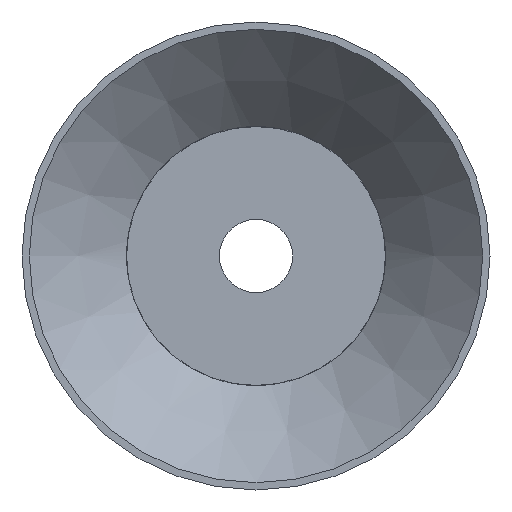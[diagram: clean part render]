
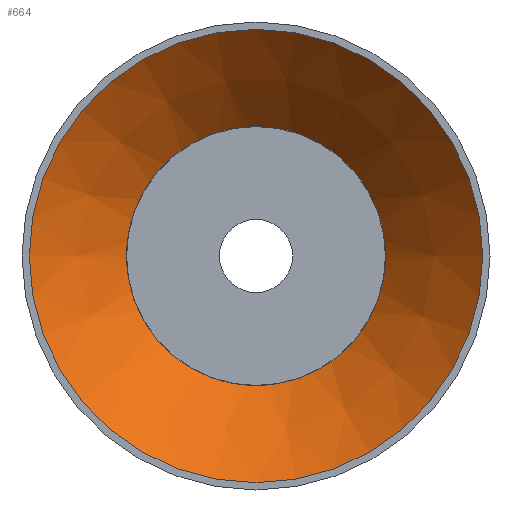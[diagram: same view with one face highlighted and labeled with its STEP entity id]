
A CAD part, front view. The second image highlights one B-rep face of the part: STEP entity #664.
In plain terms, the highlighted conical face has half-angle 43.531 degrees and reference radius 30.924 mm.
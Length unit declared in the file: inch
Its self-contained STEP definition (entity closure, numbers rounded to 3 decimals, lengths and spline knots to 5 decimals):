
#115=FACE_OUTER_BOUND('',#147,.T.);
#147=EDGE_LOOP('',(#434,#435,#436,#437,#438,#439,#440,#441,#442,#443,#444,
#445,#446));
#182=LINE('',#888,#196);
#196=VECTOR('',#768,1.2175);
#210=CIRCLE('',#711,1.55);
#211=CIRCLE('',#712,0.885);
#212=CIRCLE('',#713,0.885);
#213=CIRCLE('',#714,0.885);
#214=CIRCLE('',#715,0.885);
#215=CIRCLE('',#716,0.885);
#216=CIRCLE('',#717,0.885);
#217=CIRCLE('',#718,0.885);
#218=CIRCLE('',#719,0.885);
#219=CIRCLE('',#720,0.885);
#220=CIRCLE('',#721,1.55);
#243=VERTEX_POINT('',#884);
#244=VERTEX_POINT('',#885);
#245=VERTEX_POINT('',#887);
#246=VERTEX_POINT('',#889);
#247=VERTEX_POINT('',#891);
#248=VERTEX_POINT('',#893);
#249=VERTEX_POINT('',#895);
#250=VERTEX_POINT('',#897);
#251=VERTEX_POINT('',#899);
#252=VERTEX_POINT('',#901);
#253=VERTEX_POINT('',#903);
#320=EDGE_CURVE('',#243,#244,#210,.T.);
#321=EDGE_CURVE('',#244,#245,#182,.T.);
#322=EDGE_CURVE('',#246,#245,#211,.T.);
#323=EDGE_CURVE('',#247,#246,#212,.T.);
#324=EDGE_CURVE('',#248,#247,#213,.T.);
#325=EDGE_CURVE('',#249,#248,#214,.T.);
#326=EDGE_CURVE('',#250,#249,#215,.T.);
#327=EDGE_CURVE('',#251,#250,#216,.T.);
#328=EDGE_CURVE('',#252,#251,#217,.T.);
#329=EDGE_CURVE('',#253,#252,#218,.T.);
#330=EDGE_CURVE('',#245,#253,#219,.T.);
#331=EDGE_CURVE('',#244,#243,#220,.T.);
#434=ORIENTED_EDGE('',*,*,#320,.T.);
#435=ORIENTED_EDGE('',*,*,#321,.T.);
#436=ORIENTED_EDGE('',*,*,#322,.F.);
#437=ORIENTED_EDGE('',*,*,#323,.F.);
#438=ORIENTED_EDGE('',*,*,#324,.F.);
#439=ORIENTED_EDGE('',*,*,#325,.F.);
#440=ORIENTED_EDGE('',*,*,#326,.F.);
#441=ORIENTED_EDGE('',*,*,#327,.F.);
#442=ORIENTED_EDGE('',*,*,#328,.F.);
#443=ORIENTED_EDGE('',*,*,#329,.F.);
#444=ORIENTED_EDGE('',*,*,#330,.F.);
#445=ORIENTED_EDGE('',*,*,#321,.F.);
#446=ORIENTED_EDGE('',*,*,#331,.T.);
#662=CONICAL_SURFACE('',#710,1.2175,0.76);
#664=ADVANCED_FACE('',(#115),#662,.F.);
#710=AXIS2_PLACEMENT_3D('',#883,#764,#765);
#711=AXIS2_PLACEMENT_3D('',#886,#766,#767);
#712=AXIS2_PLACEMENT_3D('',#890,#769,#770);
#713=AXIS2_PLACEMENT_3D('',#892,#771,#772);
#714=AXIS2_PLACEMENT_3D('',#894,#773,#774);
#715=AXIS2_PLACEMENT_3D('',#896,#775,#776);
#716=AXIS2_PLACEMENT_3D('',#898,#777,#778);
#717=AXIS2_PLACEMENT_3D('',#900,#779,#780);
#718=AXIS2_PLACEMENT_3D('',#902,#781,#782);
#719=AXIS2_PLACEMENT_3D('',#904,#783,#784);
#720=AXIS2_PLACEMENT_3D('',#905,#785,#786);
#721=AXIS2_PLACEMENT_3D('',#906,#787,#788);
#764=DIRECTION('center_axis',(0.,-1.,0.));
#765=DIRECTION('ref_axis',(1.,0.,0.));
#766=DIRECTION('center_axis',(0.,-1.,0.));
#767=DIRECTION('ref_axis',(1.,0.,0.));
#768=DIRECTION('',(0.689,0.725,0.));
#769=DIRECTION('center_axis',(0.,-1.,0.));
#770=DIRECTION('ref_axis',(1.,0.,0.));
#771=DIRECTION('center_axis',(0.,-1.,0.));
#772=DIRECTION('ref_axis',(1.,0.,0.));
#773=DIRECTION('center_axis',(0.,-1.,0.));
#774=DIRECTION('ref_axis',(1.,0.,0.));
#775=DIRECTION('center_axis',(0.,-1.,0.));
#776=DIRECTION('ref_axis',(1.,0.,0.));
#777=DIRECTION('center_axis',(0.,-1.,0.));
#778=DIRECTION('ref_axis',(1.,0.,0.));
#779=DIRECTION('center_axis',(0.,-1.,0.));
#780=DIRECTION('ref_axis',(1.,0.,0.));
#781=DIRECTION('center_axis',(0.,-1.,0.));
#782=DIRECTION('ref_axis',(1.,0.,0.));
#783=DIRECTION('center_axis',(0.,-1.,0.));
#784=DIRECTION('ref_axis',(1.,0.,0.));
#785=DIRECTION('center_axis',(0.,-1.,0.));
#786=DIRECTION('ref_axis',(1.,0.,0.));
#787=DIRECTION('center_axis',(0.,-1.,0.));
#788=DIRECTION('ref_axis',(1.,0.,0.));
#883=CARTESIAN_POINT('Origin',(0.,0.35,0.));
#884=CARTESIAN_POINT('',(1.55,0.,0.));
#885=CARTESIAN_POINT('',(-1.55,0.,0.));
#886=CARTESIAN_POINT('Origin',(0.,0.,0.));
#887=CARTESIAN_POINT('',(-0.885,0.7,0.));
#888=CARTESIAN_POINT('',(-1.2175,0.35,0.));
#889=CARTESIAN_POINT('',(-0.87933,0.7,0.1));
#890=CARTESIAN_POINT('Origin',(0.,0.7,0.));
#891=CARTESIAN_POINT('',(-0.1,0.7,0.87933));
#892=CARTESIAN_POINT('Origin',(0.,0.7,0.));
#893=CARTESIAN_POINT('',(0.1,0.7,0.87933));
#894=CARTESIAN_POINT('Origin',(0.,0.7,0.));
#895=CARTESIAN_POINT('',(0.87933,0.7,0.1));
#896=CARTESIAN_POINT('Origin',(0.,0.7,0.));
#897=CARTESIAN_POINT('',(0.87933,0.7,-0.1));
#898=CARTESIAN_POINT('Origin',(0.,0.7,0.));
#899=CARTESIAN_POINT('',(0.1,0.7,-0.87933));
#900=CARTESIAN_POINT('Origin',(0.,0.7,0.));
#901=CARTESIAN_POINT('',(-0.1,0.7,-0.87933));
#902=CARTESIAN_POINT('Origin',(0.,0.7,0.));
#903=CARTESIAN_POINT('',(-0.87933,0.7,-0.1));
#904=CARTESIAN_POINT('Origin',(0.,0.7,0.));
#905=CARTESIAN_POINT('Origin',(0.,0.7,0.));
#906=CARTESIAN_POINT('Origin',(0.,0.,0.));
